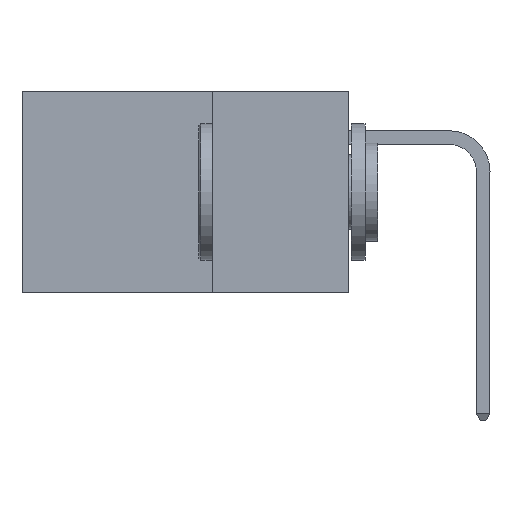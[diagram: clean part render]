
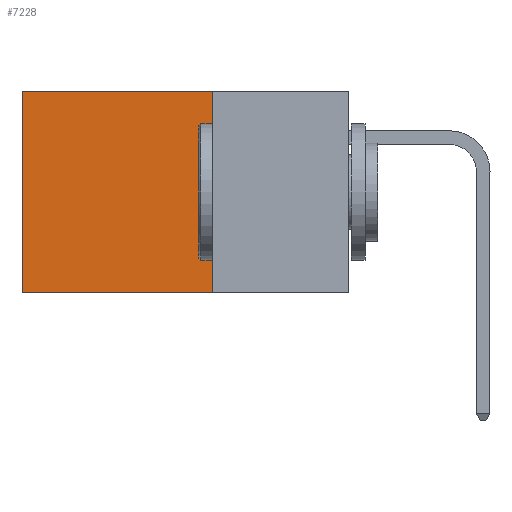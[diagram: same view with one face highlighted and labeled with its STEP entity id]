
A CAD part, left-side view. The second image highlights one B-rep face of the part: STEP entity #7228.
In plain terms, the highlighted planar face has unit normal (-1, 0, 0).
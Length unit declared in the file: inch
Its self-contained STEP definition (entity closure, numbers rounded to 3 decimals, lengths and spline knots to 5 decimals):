
#570 = VERTEX_POINT ( 'NONE', #12434 ) ;
#621 = EDGE_LOOP ( 'NONE', ( #13387, #6856, #12811, #2084 ) ) ;
#926 = DIRECTION ( 'NONE',  ( 0., 1., 0. ) ) ;
#971 = EDGE_CURVE ( 'NONE', #5827, #8040, #6090, .T. ) ;
#1072 = EDGE_CURVE ( 'NONE', #5827, #1716, #1368, .T. ) ;
#1368 = LINE ( 'NONE', #8995, #6881 ) ;
#1402 = CARTESIAN_POINT ( 'NONE',  ( 0.2875, 0.25, -0.37 ) ) ;
#1716 = VERTEX_POINT ( 'NONE', #12780 ) ;
#2084 = ORIENTED_EDGE ( 'NONE', *, *, #971, .T. ) ;
#2719 = EDGE_CURVE ( 'NONE', #8040, #570, #6193, .T. ) ;
#3424 = VECTOR ( 'NONE', #4126, 39.37008 ) ;
#3884 = VECTOR ( 'NONE', #926, 39.37008 ) ;
#3933 = CARTESIAN_POINT ( 'NONE',  ( 0.2875, 0.25, 0. ) ) ;
#4126 = DIRECTION ( 'NONE',  ( 0., 0., -1. ) ) ;
#4148 = CARTESIAN_POINT ( 'NONE',  ( 0.2875, 0.6, 0. ) ) ;
#4212 = LINE ( 'NONE', #1402, #3884 ) ;
#4261 = CARTESIAN_POINT ( 'NONE',  ( 0.2875, 0.25, 0. ) ) ;
#5291 = EDGE_CURVE ( 'NONE', #1716, #570, #4212, .T. ) ;
#5298 = DIRECTION ( 'NONE',  ( 0., 0., -1. ) ) ;
#5827 = VERTEX_POINT ( 'NONE', #3933 ) ;
#6090 = LINE ( 'NONE', #11318, #10948 ) ;
#6193 = LINE ( 'NONE', #4148, #3424 ) ;
#6753 = CARTESIAN_POINT ( 'NONE',  ( 0.2875, 0.6, 0. ) ) ;
#6856 = ORIENTED_EDGE ( 'NONE', *, *, #5291, .F. ) ;
#6881 = VECTOR ( 'NONE', #9374, 39.37008 ) ;
#7228 = ADVANCED_FACE ( 'NONE', ( #11303 ), #7326, .F. ) ;
#7326 = PLANE ( 'NONE',  #8845 ) ;
#8040 = VERTEX_POINT ( 'NONE', #6753 ) ;
#8845 = AXIS2_PLACEMENT_3D ( 'NONE', #4261, #11474, #5298 ) ;
#8995 = CARTESIAN_POINT ( 'NONE',  ( 0.2875, 0.25, 0. ) ) ;
#9374 = DIRECTION ( 'NONE',  ( 0., 0., -1. ) ) ;
#10948 = VECTOR ( 'NONE', #11252, 39.37008 ) ;
#11252 = DIRECTION ( 'NONE',  ( 0., 1., 0. ) ) ;
#11303 = FACE_OUTER_BOUND ( 'NONE', #621, .T. ) ;
#11318 = CARTESIAN_POINT ( 'NONE',  ( 0.2875, 0.25, 0. ) ) ;
#11474 = DIRECTION ( 'NONE',  ( 1., 0., 0. ) ) ;
#12434 = CARTESIAN_POINT ( 'NONE',  ( 0.2875, 0.6, -0.37 ) ) ;
#12780 = CARTESIAN_POINT ( 'NONE',  ( 0.2875, 0.25, -0.37 ) ) ;
#12811 = ORIENTED_EDGE ( 'NONE', *, *, #1072, .F. ) ;
#13387 = ORIENTED_EDGE ( 'NONE', *, *, #2719, .T. ) ;
